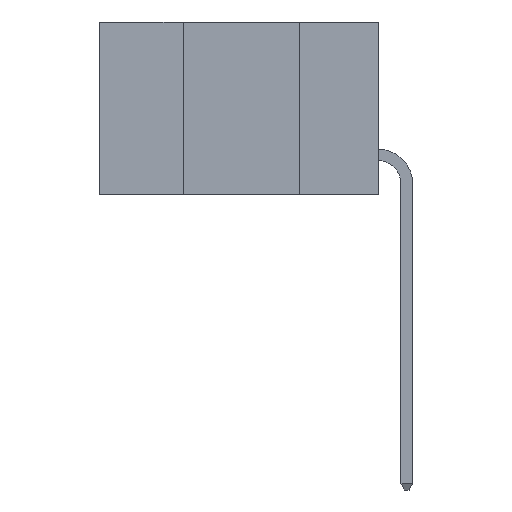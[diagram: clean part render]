
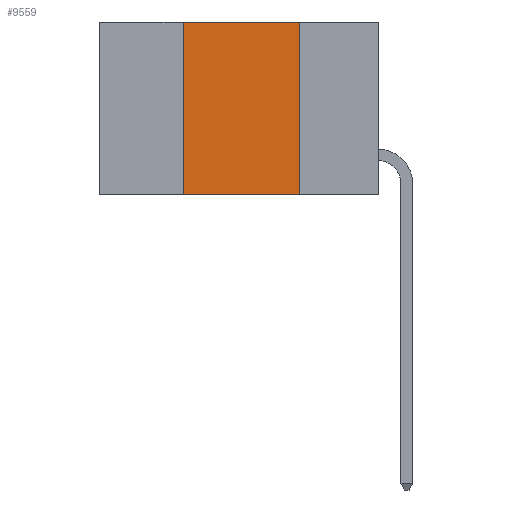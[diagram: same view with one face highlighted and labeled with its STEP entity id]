
A CAD part, left-side view. The second image highlights one B-rep face of the part: STEP entity #9559.
In plain terms, the highlighted planar face has unit normal (-1, 0, 0).
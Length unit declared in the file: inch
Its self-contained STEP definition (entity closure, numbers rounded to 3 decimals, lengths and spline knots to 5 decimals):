
#243 = VERTEX_POINT ( 'NONE', #2364 ) ;
#255 = LINE ( 'NONE', #961, #10466 ) ;
#325 = VERTEX_POINT ( 'NONE', #9835 ) ;
#348 = DIRECTION ( 'NONE',  ( 0., 0., 1. ) ) ;
#452 = CARTESIAN_POINT ( 'NONE',  ( 0., 0.42, -0.37 ) ) ;
#684 = DIRECTION ( 'NONE',  ( 0., 0., -1. ) ) ;
#961 = CARTESIAN_POINT ( 'NONE',  ( 0., 0.6, -0.37 ) ) ;
#1178 = DIRECTION ( 'NONE',  ( 0., -1., 0. ) ) ;
#1226 = CARTESIAN_POINT ( 'NONE',  ( 0., 0.6, 0. ) ) ;
#1275 = CARTESIAN_POINT ( 'NONE',  ( 0., 0.42, -0.37 ) ) ;
#1463 = FACE_OUTER_BOUND ( 'NONE', #3552, .T. ) ;
#2146 = DIRECTION ( 'NONE',  ( 0., -1., 0. ) ) ;
#2364 = CARTESIAN_POINT ( 'NONE',  ( 0., 0.42, 0. ) ) ;
#2488 = CARTESIAN_POINT ( 'NONE',  ( 0., 0.6, 0. ) ) ;
#2557 = VECTOR ( 'NONE', #684, 39.37008 ) ;
#2920 = LINE ( 'NONE', #1275, #9129 ) ;
#2946 = LINE ( 'NONE', #1226, #9156 ) ;
#3254 = CARTESIAN_POINT ( 'NONE',  ( 0., 0.17, -0.37 ) ) ;
#3298 = ORIENTED_EDGE ( 'NONE', *, *, #5706, .F. ) ;
#3305 = DIRECTION ( 'NONE',  ( 0., 0., -1. ) ) ;
#3361 = EDGE_CURVE ( 'NONE', #5793, #325, #255, .T. ) ;
#3552 = EDGE_LOOP ( 'NONE', ( #6373, #3298, #4370, #5506 ) ) ;
#4370 = ORIENTED_EDGE ( 'NONE', *, *, #8666, .F. ) ;
#4766 = LINE ( 'NONE', #3254, #2557 ) ;
#4954 = PLANE ( 'NONE',  #6608 ) ;
#5506 = ORIENTED_EDGE ( 'NONE', *, *, #3361, .T. ) ;
#5564 = CARTESIAN_POINT ( 'NONE',  ( 0., 0.17, 0. ) ) ;
#5706 = EDGE_CURVE ( 'NONE', #243, #6840, #2946, .T. ) ;
#5793 = VERTEX_POINT ( 'NONE', #452 ) ;
#5920 = EDGE_CURVE ( 'NONE', #6840, #325, #4766, .T. ) ;
#6373 = ORIENTED_EDGE ( 'NONE', *, *, #5920, .F. ) ;
#6608 = AXIS2_PLACEMENT_3D ( 'NONE', #2488, #8192, #3305 ) ;
#6840 = VERTEX_POINT ( 'NONE', #5564 ) ;
#8192 = DIRECTION ( 'NONE',  ( 1., 0., 0. ) ) ;
#8666 = EDGE_CURVE ( 'NONE', #5793, #243, #2920, .T. ) ;
#9129 = VECTOR ( 'NONE', #348, 39.37008 ) ;
#9156 = VECTOR ( 'NONE', #2146, 39.37008 ) ;
#9559 = ADVANCED_FACE ( 'NONE', ( #1463 ), #4954, .F. ) ;
#9835 = CARTESIAN_POINT ( 'NONE',  ( 0., 0.17, -0.37 ) ) ;
#10466 = VECTOR ( 'NONE', #1178, 39.37008 ) ;
